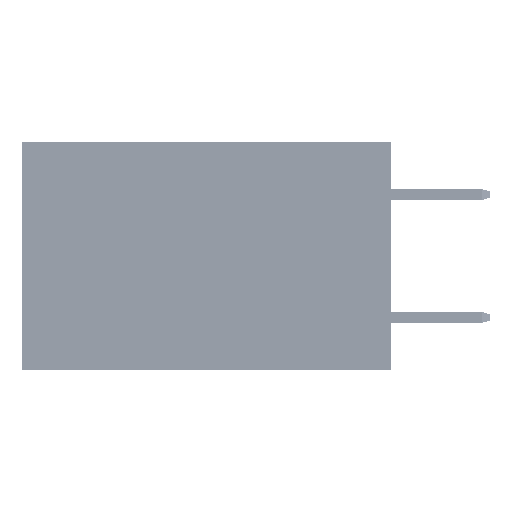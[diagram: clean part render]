
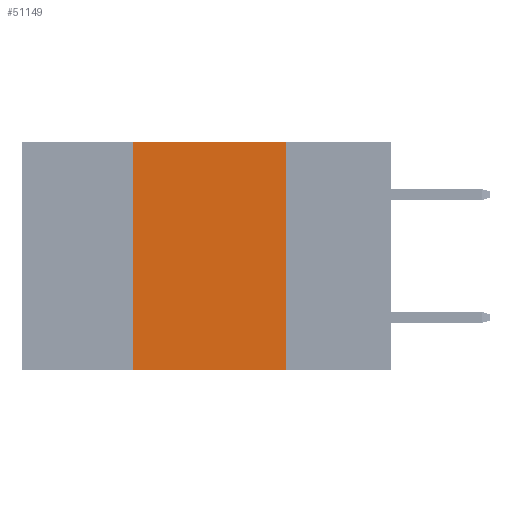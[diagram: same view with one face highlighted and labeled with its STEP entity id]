
A CAD part, left-side view. The second image highlights one B-rep face of the part: STEP entity #51149.
In plain terms, the highlighted planar face has unit normal (-1, 0, 0).
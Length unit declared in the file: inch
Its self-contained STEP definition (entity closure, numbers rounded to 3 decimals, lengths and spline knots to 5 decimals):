
#881 = EDGE_CURVE ( 'NONE', #37296, #19208, #41992, .T. ) ;
#962 = EDGE_CURVE ( 'NONE', #15504, #47177, #41214, .T. ) ;
#1080 = CARTESIAN_POINT ( 'NONE',  ( 0., 0.17, 0. ) ) ;
#3885 = ORIENTED_EDGE ( 'NONE', *, *, #881, .F. ) ;
#4838 = DIRECTION ( 'NONE',  ( 0., -1., 0. ) ) ;
#5623 = DIRECTION ( 'NONE',  ( 0., -1., 0. ) ) ;
#7448 = EDGE_CURVE ( 'NONE', #19208, #47177, #47953, .T. ) ;
#8097 = DIRECTION ( 'NONE',  ( 1., 0., 0. ) ) ;
#8360 = DIRECTION ( 'NONE',  ( 0., 0., -1. ) ) ;
#12792 = VECTOR ( 'NONE', #27776, 39.37008 ) ;
#15504 = VERTEX_POINT ( 'NONE', #46574 ) ;
#17995 = ORIENTED_EDGE ( 'NONE', *, *, #33425, .F. ) ;
#19208 = VERTEX_POINT ( 'NONE', #1080 ) ;
#21485 = ORIENTED_EDGE ( 'NONE', *, *, #7448, .F. ) ;
#24137 = EDGE_LOOP ( 'NONE', ( #21485, #3885, #17995, #48950 ) ) ;
#25166 = CARTESIAN_POINT ( 'NONE',  ( 0., 0.42, 0. ) ) ;
#27249 = CARTESIAN_POINT ( 'NONE',  ( 0., 0.17, 0. ) ) ;
#27584 = CARTESIAN_POINT ( 'NONE',  ( 0., 0.17, -0.37 ) ) ;
#27776 = DIRECTION ( 'NONE',  ( 0., 0., -1. ) ) ;
#29682 = LINE ( 'NONE', #25166, #30684 ) ;
#29789 = CARTESIAN_POINT ( 'NONE',  ( 0., 0.6, -0.37 ) ) ;
#30600 = VECTOR ( 'NONE', #4838, 39.37008 ) ;
#30684 = VECTOR ( 'NONE', #41369, 39.37008 ) ;
#31126 = AXIS2_PLACEMENT_3D ( 'NONE', #44482, #8097, #8360 ) ;
#32784 = FACE_OUTER_BOUND ( 'NONE', #24137, .T. ) ;
#33425 = EDGE_CURVE ( 'NONE', #15504, #37296, #29682, .T. ) ;
#33499 = CARTESIAN_POINT ( 'NONE',  ( 0., 0.6, 0. ) ) ;
#34765 = VECTOR ( 'NONE', #5623, 39.37008 ) ;
#37296 = VERTEX_POINT ( 'NONE', #47334 ) ;
#41214 = LINE ( 'NONE', #29789, #30600 ) ;
#41369 = DIRECTION ( 'NONE',  ( 0., 0., 1. ) ) ;
#41992 = LINE ( 'NONE', #33499, #34765 ) ;
#44482 = CARTESIAN_POINT ( 'NONE',  ( 0., 0.6, 0. ) ) ;
#46574 = CARTESIAN_POINT ( 'NONE',  ( 0., 0.42, -0.37 ) ) ;
#47177 = VERTEX_POINT ( 'NONE', #27584 ) ;
#47334 = CARTESIAN_POINT ( 'NONE',  ( 0., 0.42, 0. ) ) ;
#47953 = LINE ( 'NONE', #27249, #12792 ) ;
#48734 = PLANE ( 'NONE',  #31126 ) ;
#48950 = ORIENTED_EDGE ( 'NONE', *, *, #962, .T. ) ;
#51149 = ADVANCED_FACE ( 'NONE', ( #32784 ), #48734, .F. ) ;
